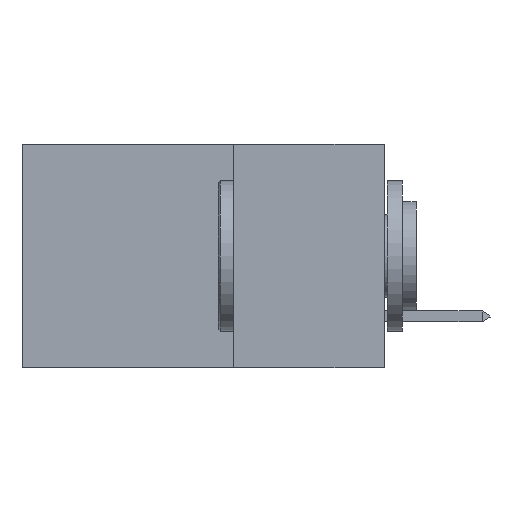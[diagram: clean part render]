
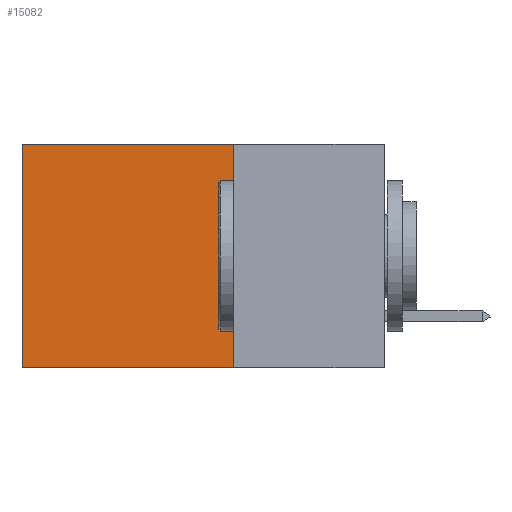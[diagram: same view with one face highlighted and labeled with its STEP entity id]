
A CAD part, left-side view. The second image highlights one B-rep face of the part: STEP entity #15082.
In plain terms, the highlighted planar face has unit normal (-1, 0, 0).
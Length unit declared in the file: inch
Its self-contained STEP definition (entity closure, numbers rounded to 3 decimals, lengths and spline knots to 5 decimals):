
#225 = LINE ( 'NONE', #8392, #12245 ) ;
#1806 = CARTESIAN_POINT ( 'NONE',  ( 0.2875, 0.25, 0. ) ) ;
#2181 = LINE ( 'NONE', #5729, #10024 ) ;
#2390 = AXIS2_PLACEMENT_3D ( 'NONE', #1806, #10019, #5384 ) ;
#3070 = VERTEX_POINT ( 'NONE', #3258 ) ;
#3258 = CARTESIAN_POINT ( 'NONE',  ( 0.2875, 0.6, 0. ) ) ;
#3360 = DIRECTION ( 'NONE',  ( 0., 0., -1. ) ) ;
#3524 = LINE ( 'NONE', #12586, #6266 ) ;
#4458 = CARTESIAN_POINT ( 'NONE',  ( 0.2875, 0.25, -0.37 ) ) ;
#4478 = EDGE_CURVE ( 'NONE', #6500, #5704, #225, .T. ) ;
#5384 = DIRECTION ( 'NONE',  ( 0., 0., -1. ) ) ;
#5559 = EDGE_CURVE ( 'NONE', #3070, #5871, #2181, .T. ) ;
#5704 = VERTEX_POINT ( 'NONE', #4458 ) ;
#5729 = CARTESIAN_POINT ( 'NONE',  ( 0.2875, 0.6, 0. ) ) ;
#5771 = ORIENTED_EDGE ( 'NONE', *, *, #5559, .T. ) ;
#5837 = CARTESIAN_POINT ( 'NONE',  ( 0.2875, 0.25, 0. ) ) ;
#5871 = VERTEX_POINT ( 'NONE', #14525 ) ;
#6266 = VECTOR ( 'NONE', #12528, 39.37008 ) ;
#6500 = VERTEX_POINT ( 'NONE', #7271 ) ;
#7271 = CARTESIAN_POINT ( 'NONE',  ( 0.2875, 0.25, 0. ) ) ;
#7755 = PLANE ( 'NONE',  #2390 ) ;
#8392 = CARTESIAN_POINT ( 'NONE',  ( 0.2875, 0.25, 0. ) ) ;
#8504 = EDGE_LOOP ( 'NONE', ( #5771, #9795, #12751, #11599 ) ) ;
#9795 = ORIENTED_EDGE ( 'NONE', *, *, #14812, .F. ) ;
#10019 = DIRECTION ( 'NONE',  ( 1., 0., 0. ) ) ;
#10023 = LINE ( 'NONE', #5837, #10553 ) ;
#10024 = VECTOR ( 'NONE', #3360, 39.37008 ) ;
#10359 = DIRECTION ( 'NONE',  ( 0., 1., 0. ) ) ;
#10553 = VECTOR ( 'NONE', #10359, 39.37008 ) ;
#10575 = FACE_OUTER_BOUND ( 'NONE', #8504, .T. ) ;
#10715 = DIRECTION ( 'NONE',  ( 0., 0., -1. ) ) ;
#11599 = ORIENTED_EDGE ( 'NONE', *, *, #12797, .T. ) ;
#12245 = VECTOR ( 'NONE', #10715, 39.37008 ) ;
#12528 = DIRECTION ( 'NONE',  ( 0., 1., 0. ) ) ;
#12586 = CARTESIAN_POINT ( 'NONE',  ( 0.2875, 0.25, -0.37 ) ) ;
#12751 = ORIENTED_EDGE ( 'NONE', *, *, #4478, .F. ) ;
#12797 = EDGE_CURVE ( 'NONE', #6500, #3070, #10023, .T. ) ;
#14525 = CARTESIAN_POINT ( 'NONE',  ( 0.2875, 0.6, -0.37 ) ) ;
#14812 = EDGE_CURVE ( 'NONE', #5704, #5871, #3524, .T. ) ;
#15082 = ADVANCED_FACE ( 'NONE', ( #10575 ), #7755, .F. ) ;
